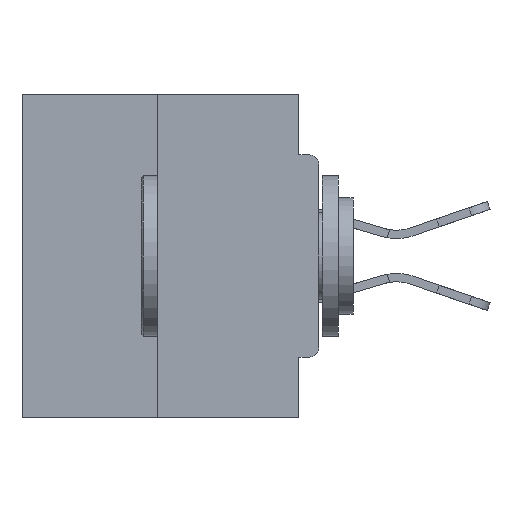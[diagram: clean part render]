
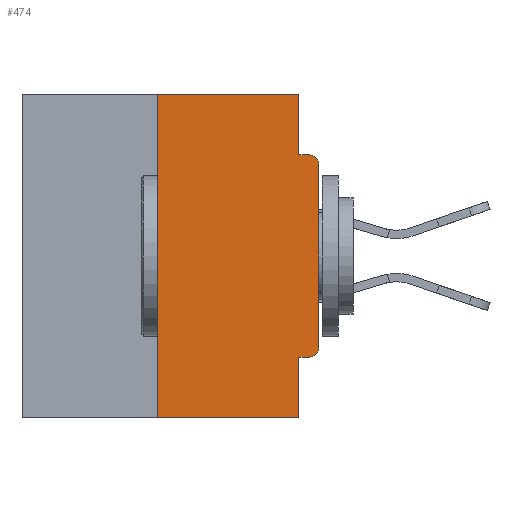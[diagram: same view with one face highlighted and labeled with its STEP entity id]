
A CAD part, left-side view. The second image highlights one B-rep face of the part: STEP entity #474.
In plain terms, the highlighted planar face has unit normal (-1, 0, 0).
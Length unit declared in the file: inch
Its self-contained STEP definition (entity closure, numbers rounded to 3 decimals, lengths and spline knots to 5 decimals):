
#265 = CARTESIAN_POINT ( 'NONE',  ( 0., 0.031, 0. ) ) ;
#474 = ADVANCED_FACE ( 'NONE', ( #7245 ), #4422, .F. ) ;
#667 = LINE ( 'NONE', #27275, #3373 ) ;
#939 = DIRECTION ( 'NONE',  ( 0., 0., -1. ) ) ;
#2401 = ORIENTED_EDGE ( 'NONE', *, *, #25944, .T. ) ;
#3344 = LINE ( 'NONE', #4813, #41556 ) ;
#3373 = VECTOR ( 'NONE', #30786, 39.37008 ) ;
#4422 = PLANE ( 'NONE',  #7604 ) ;
#4813 = CARTESIAN_POINT ( 'NONE',  ( 0., 0.46, -0.5 ) ) ;
#5526 = AXIS2_PLACEMENT_3D ( 'NONE', #6773, #31126, #20763 ) ;
#5873 = LINE ( 'NONE', #22609, #8604 ) ;
#6139 = VECTOR ( 'NONE', #33314, 39.37008 ) ;
#6199 = VECTOR ( 'NONE', #9055, 39.37008 ) ;
#6259 = CARTESIAN_POINT ( 'NONE',  ( 0., 0., -0.1085 ) ) ;
#6773 = CARTESIAN_POINT ( 'NONE',  ( 0., 0.015, -0.1085 ) ) ;
#7245 = FACE_OUTER_BOUND ( 'NONE', #15659, .T. ) ;
#7355 = ORIENTED_EDGE ( 'NONE', *, *, #22559, .F. ) ;
#7604 = AXIS2_PLACEMENT_3D ( 'NONE', #11276, #21784, #939 ) ;
#8604 = VECTOR ( 'NONE', #40345, 39.37008 ) ;
#8616 = CARTESIAN_POINT ( 'NONE',  ( 0., 0.031, -0.5 ) ) ;
#9055 = DIRECTION ( 'NONE',  ( 0., 0., -1. ) ) ;
#9171 = VERTEX_POINT ( 'NONE', #13802 ) ;
#10761 = DIRECTION ( 'NONE',  ( 0., 0., -1. ) ) ;
#11276 = CARTESIAN_POINT ( 'NONE',  ( 0., 0.46, 0. ) ) ;
#11410 = LINE ( 'NONE', #29364, #40353 ) ;
#12011 = CARTESIAN_POINT ( 'NONE',  ( 0., 0., -0.4065 ) ) ;
#12990 = CARTESIAN_POINT ( 'NONE',  ( 0., 0.015, -0.4065 ) ) ;
#13693 = LINE ( 'NONE', #265, #37151 ) ;
#13802 = CARTESIAN_POINT ( 'NONE',  ( 0., 0., -0.3915 ) ) ;
#14598 = VERTEX_POINT ( 'NONE', #15488 ) ;
#14702 = ORIENTED_EDGE ( 'NONE', *, *, #28450, .T. ) ;
#15128 = VERTEX_POINT ( 'NONE', #38511 ) ;
#15187 = DIRECTION ( 'NONE',  ( 0., 0., 1. ) ) ;
#15488 = CARTESIAN_POINT ( 'NONE',  ( 0., 0.031, -0.4065 ) ) ;
#15659 = EDGE_LOOP ( 'NONE', ( #16875, #42020, #17321, #25369, #7355, #2401, #14702, #18587, #43605, #20933 ) ) ;
#16875 = ORIENTED_EDGE ( 'NONE', *, *, #20174, .F. ) ;
#17271 = EDGE_CURVE ( 'NONE', #15128, #44707, #3344, .T. ) ;
#17321 = ORIENTED_EDGE ( 'NONE', *, *, #17271, .T. ) ;
#17801 = VERTEX_POINT ( 'NONE', #18763 ) ;
#17859 = DIRECTION ( 'NONE',  ( 0., -1., 0. ) ) ;
#18107 = LINE ( 'NONE', #8616, #6199 ) ;
#18587 = ORIENTED_EDGE ( 'NONE', *, *, #44812, .T. ) ;
#18763 = CARTESIAN_POINT ( 'NONE',  ( 0., 0.25, 0. ) ) ;
#18815 = DIRECTION ( 'NONE',  ( 0., -1., 0. ) ) ;
#19123 = LINE ( 'NONE', #21388, #35518 ) ;
#20174 = EDGE_CURVE ( 'NONE', #17801, #22484, #5873, .T. ) ;
#20763 = DIRECTION ( 'NONE',  ( 0., 0., -1. ) ) ;
#20933 = ORIENTED_EDGE ( 'NONE', *, *, #44265, .F. ) ;
#21388 = CARTESIAN_POINT ( 'NONE',  ( 0., 0., -0.0935 ) ) ;
#21779 = AXIS2_PLACEMENT_3D ( 'NONE', #33644, #30290, #33949 ) ;
#21784 = DIRECTION ( 'NONE',  ( 1., 0., 0. ) ) ;
#22484 = VERTEX_POINT ( 'NONE', #28613 ) ;
#22559 = EDGE_CURVE ( 'NONE', #27331, #14598, #37779, .T. ) ;
#22609 = CARTESIAN_POINT ( 'NONE',  ( 0., 0.46, 0. ) ) ;
#22694 = CIRCLE ( 'NONE', #21779, 0.015 ) ;
#23649 = CARTESIAN_POINT ( 'NONE',  ( 0., 0.031, -0.5 ) ) ;
#25369 = ORIENTED_EDGE ( 'NONE', *, *, #37123, .F. ) ;
#25944 = EDGE_CURVE ( 'NONE', #27331, #9171, #22694, .T. ) ;
#26561 = CARTESIAN_POINT ( 'NONE',  ( 0., 0.031, -0.0935 ) ) ;
#27221 = CIRCLE ( 'NONE', #5526, 0.015 ) ;
#27275 = CARTESIAN_POINT ( 'NONE',  ( 0., 0., 0. ) ) ;
#27331 = VERTEX_POINT ( 'NONE', #12990 ) ;
#28450 = EDGE_CURVE ( 'NONE', #9171, #37475, #667, .T. ) ;
#28462 = CARTESIAN_POINT ( 'NONE',  ( 0., 0.015, -0.0935 ) ) ;
#28613 = CARTESIAN_POINT ( 'NONE',  ( 0., 0.031, 0. ) ) ;
#29364 = CARTESIAN_POINT ( 'NONE',  ( 0., 0.25, 0. ) ) ;
#30290 = DIRECTION ( 'NONE',  ( -1., 0., 0. ) ) ;
#30786 = DIRECTION ( 'NONE',  ( 0., 0., 1. ) ) ;
#31126 = DIRECTION ( 'NONE',  ( -1., 0., 0. ) ) ;
#32021 = VERTEX_POINT ( 'NONE', #28462 ) ;
#33217 = EDGE_CURVE ( 'NONE', #33936, #32021, #19123, .T. ) ;
#33314 = DIRECTION ( 'NONE',  ( 0., 1., 0. ) ) ;
#33644 = CARTESIAN_POINT ( 'NONE',  ( 0., 0.015, -0.3915 ) ) ;
#33936 = VERTEX_POINT ( 'NONE', #26561 ) ;
#33949 = DIRECTION ( 'NONE',  ( 0., 0., -1. ) ) ;
#35518 = VECTOR ( 'NONE', #17859, 39.37008 ) ;
#37123 = EDGE_CURVE ( 'NONE', #14598, #44707, #18107, .T. ) ;
#37151 = VECTOR ( 'NONE', #10761, 39.37008 ) ;
#37475 = VERTEX_POINT ( 'NONE', #6259 ) ;
#37779 = LINE ( 'NONE', #12011, #6139 ) ;
#38511 = CARTESIAN_POINT ( 'NONE',  ( 0., 0.25, -0.5 ) ) ;
#39289 = EDGE_CURVE ( 'NONE', #15128, #17801, #11410, .T. ) ;
#40345 = DIRECTION ( 'NONE',  ( 0., -1., 0. ) ) ;
#40353 = VECTOR ( 'NONE', #15187, 39.37008 ) ;
#41556 = VECTOR ( 'NONE', #18815, 39.37008 ) ;
#42020 = ORIENTED_EDGE ( 'NONE', *, *, #39289, .F. ) ;
#43605 = ORIENTED_EDGE ( 'NONE', *, *, #33217, .F. ) ;
#44265 = EDGE_CURVE ( 'NONE', #22484, #33936, #13693, .T. ) ;
#44707 = VERTEX_POINT ( 'NONE', #23649 ) ;
#44812 = EDGE_CURVE ( 'NONE', #37475, #32021, #27221, .T. ) ;
